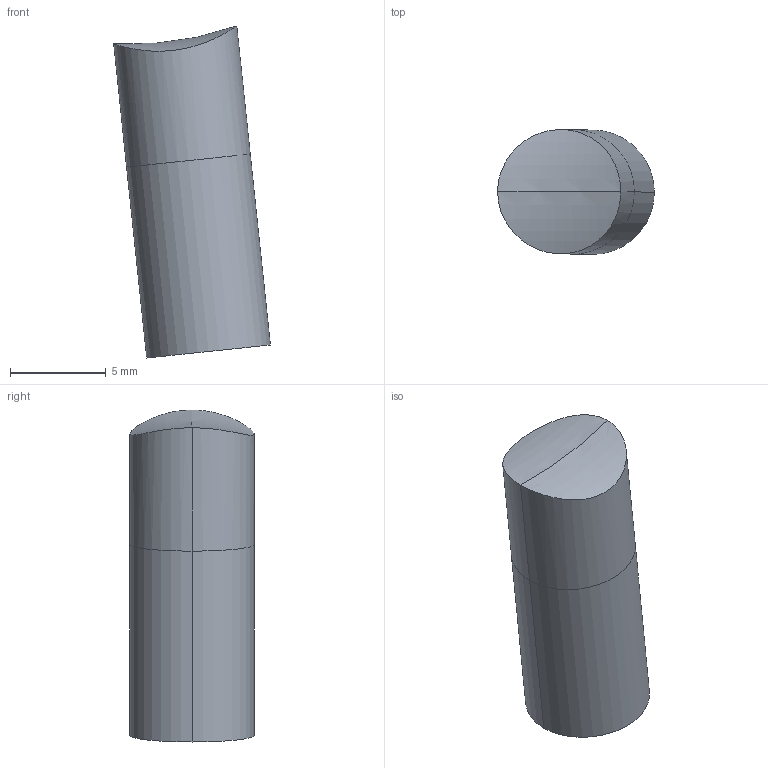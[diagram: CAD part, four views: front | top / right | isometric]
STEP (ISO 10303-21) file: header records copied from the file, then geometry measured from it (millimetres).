
FILE_DESCRIPTION (( 'STEP AP214' ), '1' );
FILE_NAME ('Buffer_Retainer_Tube_Plug.STEP', '2013-09-01T16:41:46', ( 'Asher' ), ( '' ), 'SwSTEP 2.0', 'SolidWorks 2013', '' );
FILE_SCHEMA (( 'AUTOMOTIVE_DESIGN' ));
Length unit declared in the file: millimetre
Products named in the file (1): Buffer_Retainer_Tube_Plug
Bounding box: 8.16 x 6.48 x 17.3 mm (x, y, z)
Volume: 534.7 mm3; surface area: 395.9 mm2
Topology: 1 solids, 1 shells, 7 faces, 13 edges, 8 vertices
Faces by surface type: cylinder 4, torus 2, plane 1
Entity records: 274 total; most frequent: CARTESIAN_POINT 101, DIRECTION 30, ORIENTED_EDGE 26, AXIS2_PLACEMENT_3D 13, EDGE_CURVE 13, VERTEX_POINT 8, ADVANCED_FACE 7, EDGE_LOOP 7
